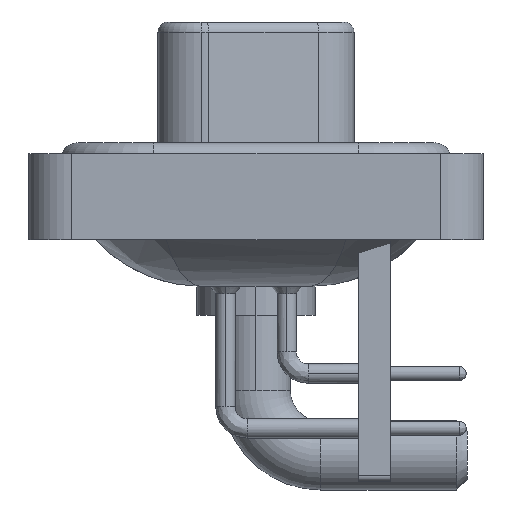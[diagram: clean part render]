
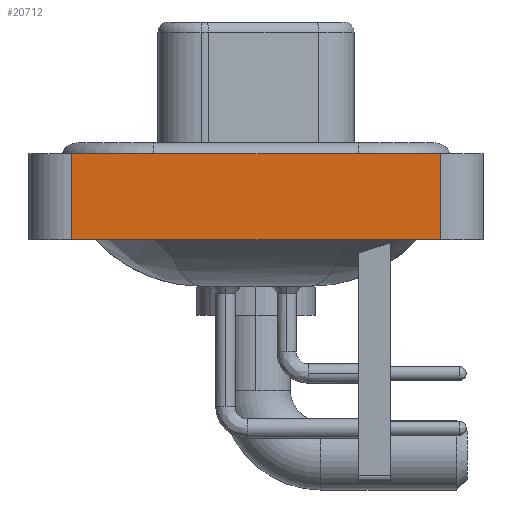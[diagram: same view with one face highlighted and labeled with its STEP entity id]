
A CAD part, left-side view. The second image highlights one B-rep face of the part: STEP entity #20712.
In plain terms, the highlighted planar face has unit normal (-1, 0, 0).
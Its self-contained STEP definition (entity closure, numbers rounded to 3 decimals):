
#280 = DIRECTION ( 'NONE',  ( -1., 0., 0. ) ) ;
#983 = VECTOR ( 'NONE', #12321, 1000. ) ;
#1232 = AXIS2_PLACEMENT_3D ( 'NONE', #16663, #280, #22265 ) ;
#1240 = DIRECTION ( 'NONE',  ( 0., -1., 0. ) ) ;
#1834 = PLANE ( 'NONE',  #1232 ) ;
#2054 = VECTOR ( 'NONE', #6165, 1000. ) ;
#2157 = LINE ( 'NONE', #11675, #12188 ) ;
#3030 = CARTESIAN_POINT ( 'NONE',  ( -7.25, -8.55, -3.6 ) ) ;
#4153 = VERTEX_POINT ( 'NONE', #23415 ) ;
#5799 = EDGE_CURVE ( 'NONE', #8220, #12106, #10776, .T. ) ;
#6165 = DIRECTION ( 'NONE',  ( 0., 0., 1. ) ) ;
#6410 = LINE ( 'NONE', #3030, #17136 ) ;
#6809 = ORIENTED_EDGE ( 'NONE', *, *, #23168, .F. ) ;
#7544 = CARTESIAN_POINT ( 'NONE',  ( -7.25, 8.55, 0.4 ) ) ;
#8220 = VERTEX_POINT ( 'NONE', #20139 ) ;
#8811 = ORIENTED_EDGE ( 'NONE', *, *, #20421, .T. ) ;
#9982 = EDGE_LOOP ( 'NONE', ( #8811, #6809, #16634, #13734 ) ) ;
#10203 = CARTESIAN_POINT ( 'NONE',  ( -7.25, -8.55, -3.6 ) ) ;
#10776 = LINE ( 'NONE', #21302, #983 ) ;
#11675 = CARTESIAN_POINT ( 'NONE',  ( -7.25, -8.55, 0.4 ) ) ;
#12106 = VERTEX_POINT ( 'NONE', #7544 ) ;
#12188 = VECTOR ( 'NONE', #16726, 1000. ) ;
#12321 = DIRECTION ( 'NONE',  ( 0., 0., 1. ) ) ;
#12697 = FACE_OUTER_BOUND ( 'NONE', #9982, .T. ) ;
#13201 = EDGE_CURVE ( 'NONE', #8220, #4153, #6410, .T. ) ;
#13734 = ORIENTED_EDGE ( 'NONE', *, *, #13201, .T. ) ;
#14300 = CARTESIAN_POINT ( 'NONE',  ( -7.25, -8.55, 0.4 ) ) ;
#16592 = VERTEX_POINT ( 'NONE', #14300 ) ;
#16634 = ORIENTED_EDGE ( 'NONE', *, *, #5799, .F. ) ;
#16663 = CARTESIAN_POINT ( 'NONE',  ( -7.25, -8.55, -3.6 ) ) ;
#16726 = DIRECTION ( 'NONE',  ( 0., -1., 0. ) ) ;
#17136 = VECTOR ( 'NONE', #1240, 1000. ) ;
#19052 = LINE ( 'NONE', #10203, #2054 ) ;
#20139 = CARTESIAN_POINT ( 'NONE',  ( -7.25, 8.55, -3.6 ) ) ;
#20421 = EDGE_CURVE ( 'NONE', #4153, #16592, #19052, .T. ) ;
#20712 = ADVANCED_FACE ( 'NONE', ( #12697 ), #1834, .T. ) ;
#21302 = CARTESIAN_POINT ( 'NONE',  ( -7.25, 8.55, -3.6 ) ) ;
#22265 = DIRECTION ( 'NONE',  ( 0., 0., 1. ) ) ;
#23168 = EDGE_CURVE ( 'NONE', #12106, #16592, #2157, .T. ) ;
#23415 = CARTESIAN_POINT ( 'NONE',  ( -7.25, -8.55, -3.6 ) ) ;
